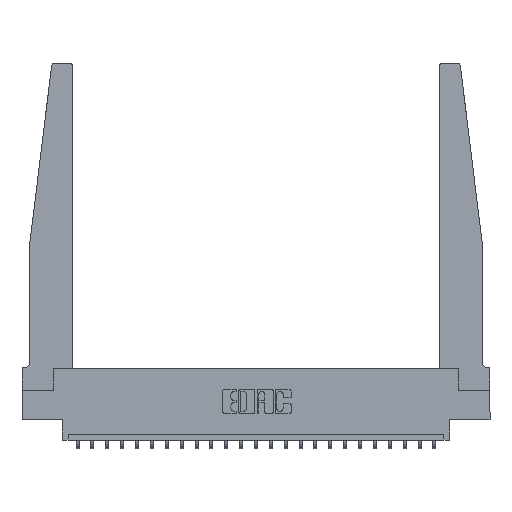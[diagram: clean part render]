
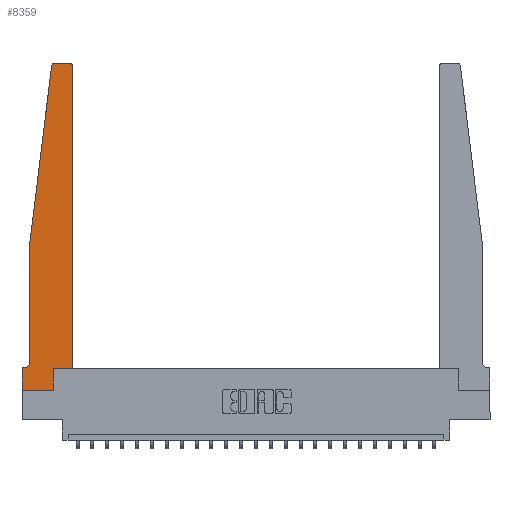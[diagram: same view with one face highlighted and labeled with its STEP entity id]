
A CAD part, top view. The second image highlights one B-rep face of the part: STEP entity #8359.
In plain terms, the highlighted planar face has unit normal (0, 0, 1).
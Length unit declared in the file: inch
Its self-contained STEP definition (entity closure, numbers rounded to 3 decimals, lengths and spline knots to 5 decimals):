
#69 = DIRECTION ( 'NONE',  ( 0., 0., 1. ) ) ;
#288 = AXIS2_PLACEMENT_3D ( 'NONE', #10645, #69, #12384 ) ;
#314 = DIRECTION ( 'NONE',  ( 1., 0., 0. ) ) ;
#718 = ORIENTED_EDGE ( 'NONE', *, *, #2961, .T. ) ;
#784 = ORIENTED_EDGE ( 'NONE', *, *, #904, .T. ) ;
#904 = EDGE_CURVE ( 'NONE', #2099, #6912, #19157, .T. ) ;
#975 = VECTOR ( 'NONE', #17282, 39.37008 ) ;
#1482 = DIRECTION ( 'NONE',  ( -0.122, -0.992, 0. ) ) ;
#1858 = ORIENTED_EDGE ( 'NONE', *, *, #2635, .T. ) ;
#2039 = LINE ( 'NONE', #2840, #11413 ) ;
#2099 = VERTEX_POINT ( 'NONE', #12211 ) ;
#2146 = ORIENTED_EDGE ( 'NONE', *, *, #18878, .T. ) ;
#2411 = LINE ( 'NONE', #18355, #7092 ) ;
#2635 = EDGE_CURVE ( 'NONE', #6491, #21702, #16910, .T. ) ;
#2840 = CARTESIAN_POINT ( 'NONE',  ( 0.065, 0.1875, 0.37 ) ) ;
#2855 = AXIS2_PLACEMENT_3D ( 'NONE', #5791, #18115, #7555 ) ;
#2873 = LINE ( 'NONE', #12631, #7556 ) ;
#2961 = EDGE_CURVE ( 'NONE', #3022, #16008, #14983, .T. ) ;
#2988 = CARTESIAN_POINT ( 'NONE',  ( 0.27653, 2.72, 0.37 ) ) ;
#3022 = VERTEX_POINT ( 'NONE', #11198 ) ;
#3552 = CARTESIAN_POINT ( 'NONE',  ( 0.425, 0.18, 0.37 ) ) ;
#3949 = VECTOR ( 'NONE', #21491, 39.37008 ) ;
#4153 = EDGE_CURVE ( 'NONE', #8507, #11664, #10526, .T. ) ;
#4756 = DIRECTION ( 'NONE',  ( 1., 0., 0. ) ) ;
#5021 = LINE ( 'NONE', #19709, #3949 ) ;
#5189 = DIRECTION ( 'NONE',  ( 0., 0., -1. ) ) ;
#5791 = CARTESIAN_POINT ( 'NONE',  ( 0.395, 2.72, 0.37 ) ) ;
#5863 = DIRECTION ( 'NONE',  ( -1., 0., 0. ) ) ;
#6491 = VERTEX_POINT ( 'NONE', #16829 ) ;
#6628 = EDGE_CURVE ( 'NONE', #16473, #3022, #18962, .T. ) ;
#6645 = CARTESIAN_POINT ( 'NONE',  ( 0.2605, 0.18, 0.37 ) ) ;
#6912 = VERTEX_POINT ( 'NONE', #8203 ) ;
#7092 = VECTOR ( 'NONE', #5863, 39.37008 ) ;
#7555 = DIRECTION ( 'NONE',  ( 1., 0., 0. ) ) ;
#7556 = VECTOR ( 'NONE', #314, 39.37008 ) ;
#8195 = ORIENTED_EDGE ( 'NONE', *, *, #9750, .T. ) ;
#8203 = CARTESIAN_POINT ( 'NONE',  ( 0.065, 0.2375, 0.37 ) ) ;
#8359 = ADVANCED_FACE ( 'NONE', ( #16418 ), #15875, .T. ) ;
#8507 = VERTEX_POINT ( 'NONE', #16259 ) ;
#8873 = EDGE_CURVE ( 'NONE', #6912, #22215, #12235, .T. ) ;
#9181 = VERTEX_POINT ( 'NONE', #21820 ) ;
#9607 = VECTOR ( 'NONE', #21478, 39.37008 ) ;
#9750 = EDGE_CURVE ( 'NONE', #9181, #22553, #5021, .T. ) ;
#10138 = ORIENTED_EDGE ( 'NONE', *, *, #18608, .T. ) ;
#10526 = CIRCLE ( 'NONE', #20431, 0.03 ) ;
#10645 = CARTESIAN_POINT ( 'NONE',  ( 0., 0.1875, 0.37 ) ) ;
#11198 = CARTESIAN_POINT ( 'NONE',  ( 0.425, 2.72, 0.37 ) ) ;
#11413 = VECTOR ( 'NONE', #15180, 39.37008 ) ;
#11664 = VERTEX_POINT ( 'NONE', #16552 ) ;
#12176 = CARTESIAN_POINT ( 'NONE',  ( 0.395, 2.75, 0.37 ) ) ;
#12211 = CARTESIAN_POINT ( 'NONE',  ( 0.065, 1.25, 0.37 ) ) ;
#12218 = VECTOR ( 'NONE', #20738, 39.37008 ) ;
#12235 = CIRCLE ( 'NONE', #14030, 0.05 ) ;
#12384 = DIRECTION ( 'NONE',  ( 1., 0., 0. ) ) ;
#12631 = CARTESIAN_POINT ( 'NONE',  ( 0., 0., 0.37 ) ) ;
#13006 = CARTESIAN_POINT ( 'NONE',  ( 0.015, 0.1875, 0.37 ) ) ;
#13137 = EDGE_CURVE ( 'NONE', #16008, #8507, #2411, .T. ) ;
#13577 = VECTOR ( 'NONE', #19506, 39.37008 ) ;
#13730 = ORIENTED_EDGE ( 'NONE', *, *, #4153, .T. ) ;
#13819 = CARTESIAN_POINT ( 'NONE',  ( 0.065, 1.25, 0.37 ) ) ;
#14030 = AXIS2_PLACEMENT_3D ( 'NONE', #15768, #5189, #17526 ) ;
#14474 = CARTESIAN_POINT ( 'NONE',  ( 0.425, 0.18, 0.37 ) ) ;
#14983 = CIRCLE ( 'NONE', #2855, 0.03 ) ;
#15180 = DIRECTION ( 'NONE',  ( -1., 0., 0. ) ) ;
#15316 = DIRECTION ( 'NONE',  ( 0., 0., 1. ) ) ;
#15768 = CARTESIAN_POINT ( 'NONE',  ( 0.015, 0.2375, 0.37 ) ) ;
#15875 = PLANE ( 'NONE',  #288 ) ;
#15957 = ORIENTED_EDGE ( 'NONE', *, *, #15967, .T. ) ;
#15967 = EDGE_CURVE ( 'NONE', #11664, #2099, #21028, .T. ) ;
#16008 = VERTEX_POINT ( 'NONE', #12176 ) ;
#16098 = EDGE_CURVE ( 'NONE', #21702, #16473, #18261, .T. ) ;
#16259 = CARTESIAN_POINT ( 'NONE',  ( 0.27653, 2.75, 0.37 ) ) ;
#16418 = FACE_OUTER_BOUND ( 'NONE', #18674, .T. ) ;
#16473 = VERTEX_POINT ( 'NONE', #3552 ) ;
#16552 = CARTESIAN_POINT ( 'NONE',  ( 0.24675, 2.72367, 0.37 ) ) ;
#16829 = CARTESIAN_POINT ( 'NONE',  ( 0.2605, 0., 0.37 ) ) ;
#16891 = VECTOR ( 'NONE', #1482, 39.37008 ) ;
#16910 = LINE ( 'NONE', #6645, #12218 ) ;
#17282 = DIRECTION ( 'NONE',  ( 0., -1., 0. ) ) ;
#17526 = DIRECTION ( 'NONE',  ( -1., 0., 0. ) ) ;
#17726 = CARTESIAN_POINT ( 'NONE',  ( 0.425, 0.18, 0.37 ) ) ;
#17795 = ORIENTED_EDGE ( 'NONE', *, *, #6628, .T. ) ;
#17991 = CARTESIAN_POINT ( 'NONE',  ( 0., 0., 0.37 ) ) ;
#18115 = DIRECTION ( 'NONE',  ( 0., 0., 1. ) ) ;
#18261 = LINE ( 'NONE', #17726, #13577 ) ;
#18355 = CARTESIAN_POINT ( 'NONE',  ( 0.25, 2.75, 0.37 ) ) ;
#18608 = EDGE_CURVE ( 'NONE', #22553, #6491, #2873, .T. ) ;
#18674 = EDGE_LOOP ( 'NONE', ( #21708, #13730, #15957, #784, #21159, #2146, #8195, #10138, #1858, #18892, #17795, #718 ) ) ;
#18725 = CARTESIAN_POINT ( 'NONE',  ( 0.2605, 0.18, 0.37 ) ) ;
#18878 = EDGE_CURVE ( 'NONE', #22215, #9181, #2039, .T. ) ;
#18892 = ORIENTED_EDGE ( 'NONE', *, *, #16098, .T. ) ;
#18962 = LINE ( 'NONE', #14474, #9607 ) ;
#19157 = LINE ( 'NONE', #20813, #975 ) ;
#19506 = DIRECTION ( 'NONE',  ( 1., 0., 0. ) ) ;
#19709 = CARTESIAN_POINT ( 'NONE',  ( 0., 0., 0.37 ) ) ;
#20431 = AXIS2_PLACEMENT_3D ( 'NONE', #2988, #15316, #4756 ) ;
#20738 = DIRECTION ( 'NONE',  ( 0., 1., 0. ) ) ;
#20813 = CARTESIAN_POINT ( 'NONE',  ( 0.065, 1.25, 0.37 ) ) ;
#21028 = LINE ( 'NONE', #13819, #16891 ) ;
#21159 = ORIENTED_EDGE ( 'NONE', *, *, #8873, .T. ) ;
#21478 = DIRECTION ( 'NONE',  ( 0., 1., 0. ) ) ;
#21491 = DIRECTION ( 'NONE',  ( 0., -1., 0. ) ) ;
#21702 = VERTEX_POINT ( 'NONE', #18725 ) ;
#21708 = ORIENTED_EDGE ( 'NONE', *, *, #13137, .T. ) ;
#21820 = CARTESIAN_POINT ( 'NONE',  ( 0., 0.1875, 0.37 ) ) ;
#22215 = VERTEX_POINT ( 'NONE', #13006 ) ;
#22553 = VERTEX_POINT ( 'NONE', #17991 ) ;
